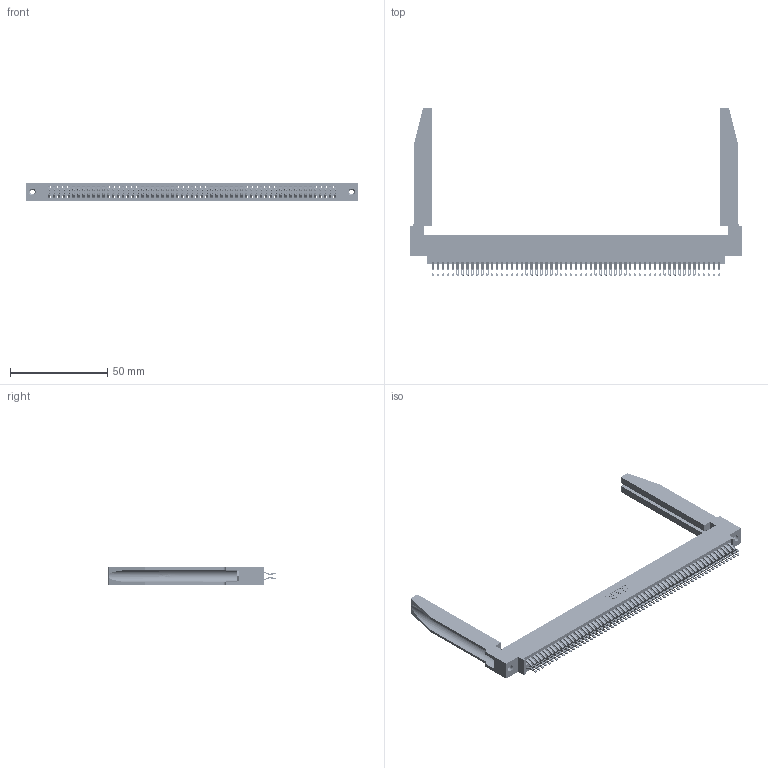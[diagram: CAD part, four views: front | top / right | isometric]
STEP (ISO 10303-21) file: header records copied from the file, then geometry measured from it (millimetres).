
FILE_DESCRIPTION (( 'STEP AP203' ), '1' );
FILE_NAME ('345-118-555-878.STEP', '2019-11-05T21:32:43', ( '' ), ( '' ), 'SwSTEP 2.0', 'SolidWorks 2016', '' );
FILE_SCHEMA (( 'CONFIG_CONTROL_DESIGN' ));
Length unit declared in the file: inch
Products named in the file (5): 345-220-078_345-220-078; 345-118-555-878; 345-292-001_555 Tail; 345-250-001_345-250-001-102; 345 Part_0.170 Offset - 0.156 Dia-TH
Assembly tree (123 placements, depth 2):
  345-118-555-878
    345 Part_0.170 Offset - 0.156 Dia-TH
    345-292-001_555 Tail  x118
    345-250-001_345-250-001-102  x2
    345-220-078_345-220-078  x2
Bounding box: 171.09 x 86.41 x 9.4 mm (x, y, z)
Volume: 24777.4 mm3; surface area: 33640.8 mm2
Topology: 123 solids, 123 shells, 6972 faces, 21847 edges, 14554 vertices
Faces by surface type: plane 3884, cylinder 3036, bspline 36, cone 12, torus 4
Entity records: 49202 total; most frequent: CARTESIAN_POINT 9185, ORIENTED_EDGE 7986, DIRECTION 7039, EDGE_CURVE 3993, VECTOR 3511, LINE 3511, VERTEX_POINT 2656, AXIS2_PLACEMENT_3D 1764
